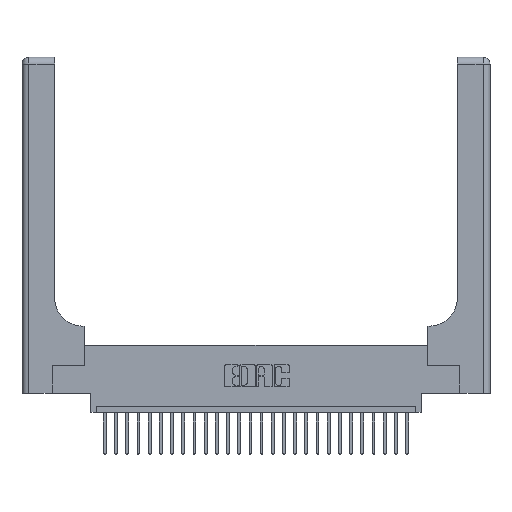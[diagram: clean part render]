
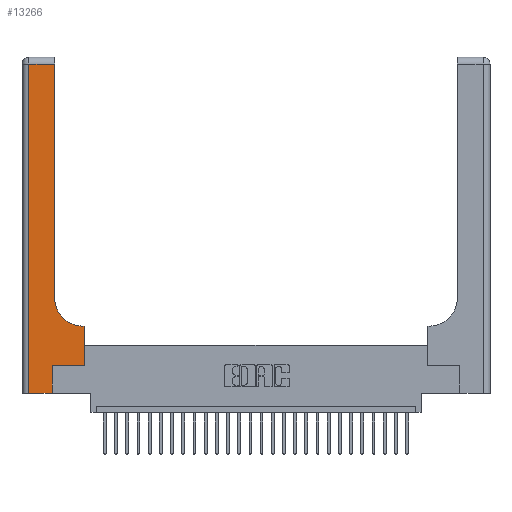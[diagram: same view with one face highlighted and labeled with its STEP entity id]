
A CAD part, top view. The second image highlights one B-rep face of the part: STEP entity #13266.
In plain terms, the highlighted planar face has unit normal (0, 0, 1).
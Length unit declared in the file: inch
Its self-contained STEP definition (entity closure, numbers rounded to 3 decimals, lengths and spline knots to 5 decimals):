
#196 = EDGE_CURVE ( 'NONE', #1369, #25235, #14174, .T. ) ;
#748 = DIRECTION ( 'NONE',  ( -1., 0., 0. ) ) ;
#1035 = VECTOR ( 'NONE', #11756, 39.37008 ) ;
#1217 = CARTESIAN_POINT ( 'NONE',  ( 0.5415, 0.6, 0.37 ) ) ;
#1369 = VERTEX_POINT ( 'NONE', #1217 ) ;
#1581 = DIRECTION ( 'NONE',  ( 0., 0., -1. ) ) ;
#1658 = CARTESIAN_POINT ( 'NONE',  ( 0.269, 0.25, 0.37 ) ) ;
#1926 = VERTEX_POINT ( 'NONE', #21173 ) ;
#2023 = CARTESIAN_POINT ( 'NONE',  ( 0.269, 0.25, 0.37 ) ) ;
#2186 = CARTESIAN_POINT ( 'NONE',  ( 0.2915, 3., 0.37 ) ) ;
#2734 = CARTESIAN_POINT ( 'NONE',  ( 0.2915, 0.6, 0.37 ) ) ;
#2789 = VERTEX_POINT ( 'NONE', #2023 ) ;
#3442 = LINE ( 'NONE', #2186, #17106 ) ;
#3801 = ORIENTED_EDGE ( 'NONE', *, *, #5770, .T. ) ;
#3934 = VECTOR ( 'NONE', #24235, 39.37008 ) ;
#3941 = DIRECTION ( 'NONE',  ( 1., 0., 0. ) ) ;
#4067 = ORIENTED_EDGE ( 'NONE', *, *, #5251, .T. ) ;
#4186 = CARTESIAN_POINT ( 'NONE',  ( 0.2915, 0.85, 0.37 ) ) ;
#4365 = LINE ( 'NONE', #5456, #26944 ) ;
#5251 = EDGE_CURVE ( 'NONE', #13192, #1369, #14571, .T. ) ;
#5288 = ORIENTED_EDGE ( 'NONE', *, *, #10795, .T. ) ;
#5456 = CARTESIAN_POINT ( 'NONE',  ( 0., 2.94, 0.37 ) ) ;
#5770 = EDGE_CURVE ( 'NONE', #12515, #1926, #25842, .T. ) ;
#5784 = LINE ( 'NONE', #10428, #22217 ) ;
#6006 = VECTOR ( 'NONE', #15815, 39.37008 ) ;
#7056 = FACE_OUTER_BOUND ( 'NONE', #8293, .T. ) ;
#7753 = DIRECTION ( 'NONE',  ( -1., 0., 0. ) ) ;
#7938 = EDGE_CURVE ( 'NONE', #16371, #13192, #22410, .T. ) ;
#7963 = CARTESIAN_POINT ( 'NONE',  ( 0.06, 0., 0.37 ) ) ;
#8293 = EDGE_LOOP ( 'NONE', ( #22808, #15904, #13839, #3801, #5288, #17848, #23111, #4067, #14451 ) ) ;
#9893 = DIRECTION ( 'NONE',  ( 0., 0., -1. ) ) ;
#10092 = VECTOR ( 'NONE', #14361, 39.37008 ) ;
#10428 = CARTESIAN_POINT ( 'NONE',  ( 0.06, 3., 0.37 ) ) ;
#10790 = VERTEX_POINT ( 'NONE', #22370 ) ;
#10795 = EDGE_CURVE ( 'NONE', #1926, #2789, #12636, .T. ) ;
#10851 = DIRECTION ( 'NONE',  ( 0., 1., 0. ) ) ;
#11756 = DIRECTION ( 'NONE',  ( 0., 1., 0. ) ) ;
#11940 = EDGE_CURVE ( 'NONE', #10790, #22936, #4365, .T. ) ;
#12515 = VERTEX_POINT ( 'NONE', #7963 ) ;
#12636 = LINE ( 'NONE', #15779, #1035 ) ;
#13192 = VERTEX_POINT ( 'NONE', #26819 ) ;
#13266 = ADVANCED_FACE ( 'NONE', ( #7056 ), #27016, .F. ) ;
#13839 = ORIENTED_EDGE ( 'NONE', *, *, #23819, .T. ) ;
#14174 = CIRCLE ( 'NONE', #14474, 0.25 ) ;
#14361 = DIRECTION ( 'NONE',  ( 0., 1., 0. ) ) ;
#14451 = ORIENTED_EDGE ( 'NONE', *, *, #196, .T. ) ;
#14474 = AXIS2_PLACEMENT_3D ( 'NONE', #17030, #1581, #3941 ) ;
#14571 = LINE ( 'NONE', #2734, #6006 ) ;
#14834 = EDGE_CURVE ( 'NONE', #25235, #10790, #3442, .T. ) ;
#15215 = EDGE_CURVE ( 'NONE', #2789, #16371, #17779, .T. ) ;
#15682 = CARTESIAN_POINT ( 'NONE',  ( 0., 0., 0.37 ) ) ;
#15779 = CARTESIAN_POINT ( 'NONE',  ( 0.269, 0., 0.37 ) ) ;
#15815 = DIRECTION ( 'NONE',  ( -1., 0., 0. ) ) ;
#15904 = ORIENTED_EDGE ( 'NONE', *, *, #11940, .T. ) ;
#16165 = AXIS2_PLACEMENT_3D ( 'NONE', #22814, #9893, #748 ) ;
#16371 = VERTEX_POINT ( 'NONE', #27916 ) ;
#17030 = CARTESIAN_POINT ( 'NONE',  ( 0.5415, 0.85, 0.37 ) ) ;
#17106 = VECTOR ( 'NONE', #10851, 39.37008 ) ;
#17779 = LINE ( 'NONE', #1658, #23607 ) ;
#17848 = ORIENTED_EDGE ( 'NONE', *, *, #15215, .T. ) ;
#18727 = DIRECTION ( 'NONE',  ( 1., 0., 0. ) ) ;
#20282 = CARTESIAN_POINT ( 'NONE',  ( 0.06, 2.94, 0.37 ) ) ;
#21173 = CARTESIAN_POINT ( 'NONE',  ( 0.269, 0., 0.37 ) ) ;
#22217 = VECTOR ( 'NONE', #27706, 39.37008 ) ;
#22370 = CARTESIAN_POINT ( 'NONE',  ( 0.2915, 2.94, 0.37 ) ) ;
#22410 = LINE ( 'NONE', #25490, #10092 ) ;
#22808 = ORIENTED_EDGE ( 'NONE', *, *, #14834, .T. ) ;
#22814 = CARTESIAN_POINT ( 'NONE',  ( 0., 3., 0.37 ) ) ;
#22936 = VERTEX_POINT ( 'NONE', #20282 ) ;
#23111 = ORIENTED_EDGE ( 'NONE', *, *, #7938, .T. ) ;
#23607 = VECTOR ( 'NONE', #18727, 39.37008 ) ;
#23819 = EDGE_CURVE ( 'NONE', #22936, #12515, #5784, .T. ) ;
#24235 = DIRECTION ( 'NONE',  ( 1., 0., 0. ) ) ;
#25235 = VERTEX_POINT ( 'NONE', #4186 ) ;
#25490 = CARTESIAN_POINT ( 'NONE',  ( 0.5585, 0.25, 0.37 ) ) ;
#25842 = LINE ( 'NONE', #15682, #3934 ) ;
#26819 = CARTESIAN_POINT ( 'NONE',  ( 0.5585, 0.6, 0.37 ) ) ;
#26944 = VECTOR ( 'NONE', #7753, 39.37008 ) ;
#27016 = PLANE ( 'NONE',  #16165 ) ;
#27706 = DIRECTION ( 'NONE',  ( 0., -1., 0. ) ) ;
#27916 = CARTESIAN_POINT ( 'NONE',  ( 0.5585, 0.25, 0.37 ) ) ;
